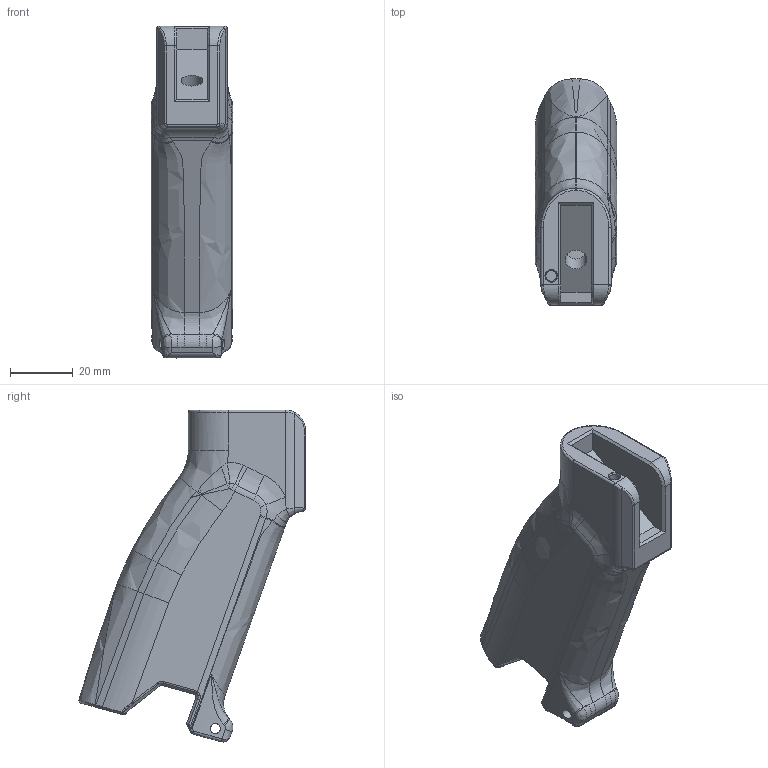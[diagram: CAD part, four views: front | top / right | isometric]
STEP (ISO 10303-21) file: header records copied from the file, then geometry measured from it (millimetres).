
FILE_DESCRIPTION(/* description */ (''),/* implementation_level */ '2;1');
FILE_NAME(/* name */ 'Standard Grip Body.step',/* time_stamp */ '2021-05-07T03:06:22-04:00',/* author */ (''),/* organization */ (''),/* preprocessor_version */ 'ST-DEVELOPER v18.1',/* originating_system */ 'Autodesk Translation Framework v10.6.0.1341',/* authorisation */ '');
FILE_SCHEMA (('AUTOMOTIVE_DESIGN { 1 0 10303 214 3 1 1 }'));
Length unit declared in the file: millimetre
Products named in the file (1): Standard Grip Body
Bounding box: 25.93 x 72.09 x 105.63 mm (x, y, z)
Volume: 41249.1 mm3; surface area: 22137.3 mm2
Topology: 1 solids, 1 shells, 470 faces, 1166 edges, 681 vertices
Faces by surface type: bspline 288, plane 80, cylinder 71, torus 17, cone 12, sphere 2
Full cylindrical faces by diameter (mm): 3.2 x2, 3.4 x1, 6.8 x1
Entity records: 21998 total; most frequent: CARTESIAN_POINT 12816, ORIENTED_EDGE 2296, DIRECTION 1232, EDGE_CURVE 1148, VERTEX_POINT 681, B_SPLINE_CURVE_WITH_KNOTS 566, EDGE_LOOP 477, FACE_OUTER_BOUND 470
